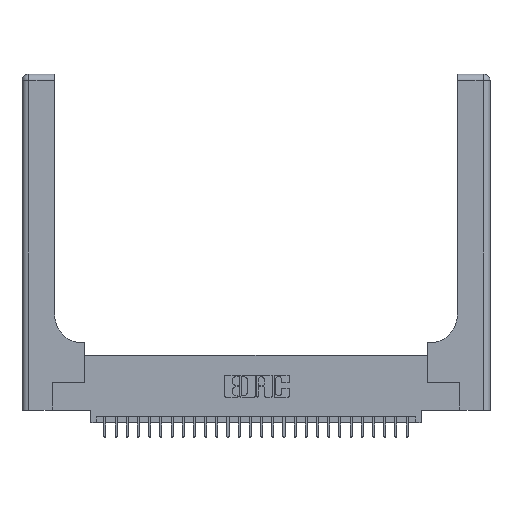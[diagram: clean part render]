
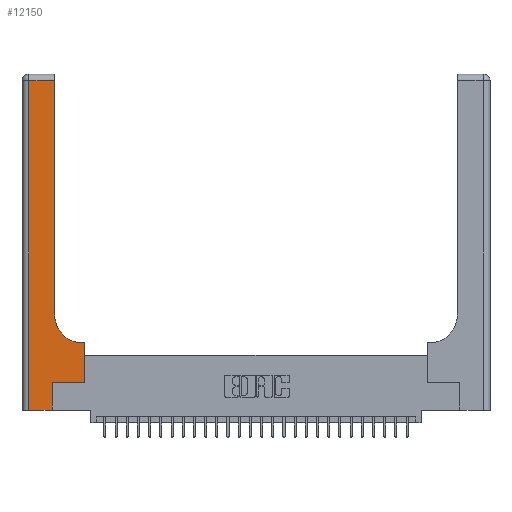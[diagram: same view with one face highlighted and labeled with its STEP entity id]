
A CAD part, top view. The second image highlights one B-rep face of the part: STEP entity #12150.
In plain terms, the highlighted planar face has unit normal (0, 0, 1).
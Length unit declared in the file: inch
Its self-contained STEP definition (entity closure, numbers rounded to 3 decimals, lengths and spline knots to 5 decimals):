
#616 = VECTOR ( 'NONE', #13172, 39.37008 ) ;
#1050 = CARTESIAN_POINT ( 'NONE',  ( 0.5585, 0.25, 0.37 ) ) ;
#1435 = AXIS2_PLACEMENT_3D ( 'NONE', #8181, #15142, #17243 ) ;
#1780 = FACE_OUTER_BOUND ( 'NONE', #25317, .T. ) ;
#2160 = DIRECTION ( 'NONE',  ( 0., 1., 0. ) ) ;
#2464 = VECTOR ( 'NONE', #2160, 39.37008 ) ;
#3300 = LINE ( 'NONE', #1050, #7181 ) ;
#3573 = CARTESIAN_POINT ( 'NONE',  ( 0.2915, 2.94, 0.37 ) ) ;
#4096 = EDGE_CURVE ( 'NONE', #13927, #12521, #15370, .T. ) ;
#4143 = CARTESIAN_POINT ( 'NONE',  ( 0., 0., 0.37 ) ) ;
#4147 = VECTOR ( 'NONE', #22045, 39.37008 ) ;
#4674 = ORIENTED_EDGE ( 'NONE', *, *, #13537, .T. ) ;
#5529 = EDGE_CURVE ( 'NONE', #14583, #12405, #22468, .T. ) ;
#5566 = ORIENTED_EDGE ( 'NONE', *, *, #5529, .T. ) ;
#5905 = DIRECTION ( 'NONE',  ( 1., 0., 0. ) ) ;
#6314 = CARTESIAN_POINT ( 'NONE',  ( 0.269, 0., 0.37 ) ) ;
#6550 = CIRCLE ( 'NONE', #19799, 0.25 ) ;
#7181 = VECTOR ( 'NONE', #7725, 39.37008 ) ;
#7462 = CARTESIAN_POINT ( 'NONE',  ( 0.06, 2.94, 0.37 ) ) ;
#7725 = DIRECTION ( 'NONE',  ( 0., 1., 0. ) ) ;
#7911 = EDGE_CURVE ( 'NONE', #12521, #24864, #22791, .T. ) ;
#8181 = CARTESIAN_POINT ( 'NONE',  ( 0., 3., 0.37 ) ) ;
#9053 = CARTESIAN_POINT ( 'NONE',  ( 0.5415, 0.6, 0.37 ) ) ;
#10012 = EDGE_CURVE ( 'NONE', #28641, #14583, #15413, .T. ) ;
#10838 = PLANE ( 'NONE',  #1435 ) ;
#10984 = VECTOR ( 'NONE', #22379, 39.37008 ) ;
#10993 = CARTESIAN_POINT ( 'NONE',  ( 0.5585, 0.6, 0.37 ) ) ;
#11011 = VERTEX_POINT ( 'NONE', #22078 ) ;
#11362 = DIRECTION ( 'NONE',  ( -1., 0., 0. ) ) ;
#11471 = VECTOR ( 'NONE', #11362, 39.37008 ) ;
#11525 = CARTESIAN_POINT ( 'NONE',  ( 0.2915, 3., 0.37 ) ) ;
#12150 = ADVANCED_FACE ( 'NONE', ( #1780 ), #10838, .F. ) ;
#12405 = VERTEX_POINT ( 'NONE', #23147 ) ;
#12521 = VERTEX_POINT ( 'NONE', #3573 ) ;
#12564 = CARTESIAN_POINT ( 'NONE',  ( 0.5415, 0.85, 0.37 ) ) ;
#12639 = ORIENTED_EDGE ( 'NONE', *, *, #16860, .T. ) ;
#13126 = CARTESIAN_POINT ( 'NONE',  ( 0.269, 0.25, 0.37 ) ) ;
#13148 = ORIENTED_EDGE ( 'NONE', *, *, #21760, .T. ) ;
#13172 = DIRECTION ( 'NONE',  ( 1., 0., 0. ) ) ;
#13273 = LINE ( 'NONE', #13126, #4147 ) ;
#13344 = VERTEX_POINT ( 'NONE', #9053 ) ;
#13370 = VERTEX_POINT ( 'NONE', #10993 ) ;
#13537 = EDGE_CURVE ( 'NONE', #11011, #13370, #3300, .T. ) ;
#13927 = VERTEX_POINT ( 'NONE', #29030 ) ;
#14583 = VERTEX_POINT ( 'NONE', #22043 ) ;
#15142 = DIRECTION ( 'NONE',  ( 0., 0., -1. ) ) ;
#15370 = LINE ( 'NONE', #11525, #24630 ) ;
#15413 = LINE ( 'NONE', #4143, #616 ) ;
#15873 = VECTOR ( 'NONE', #18254, 39.37008 ) ;
#16011 = CARTESIAN_POINT ( 'NONE',  ( 0.06, 3., 0.37 ) ) ;
#16860 = EDGE_CURVE ( 'NONE', #13370, #13344, #27652, .T. ) ;
#17243 = DIRECTION ( 'NONE',  ( -1., 0., 0. ) ) ;
#17843 = ORIENTED_EDGE ( 'NONE', *, *, #24388, .T. ) ;
#18054 = CARTESIAN_POINT ( 'NONE',  ( 0., 2.94, 0.37 ) ) ;
#18254 = DIRECTION ( 'NONE',  ( 0., -1., 0. ) ) ;
#19799 = AXIS2_PLACEMENT_3D ( 'NONE', #12564, #21614, #5905 ) ;
#20201 = ORIENTED_EDGE ( 'NONE', *, *, #10012, .T. ) ;
#21292 = CARTESIAN_POINT ( 'NONE',  ( 0.06, 0., 0.37 ) ) ;
#21614 = DIRECTION ( 'NONE',  ( 0., 0., -1. ) ) ;
#21760 = EDGE_CURVE ( 'NONE', #24864, #28641, #25211, .T. ) ;
#22043 = CARTESIAN_POINT ( 'NONE',  ( 0.269, 0., 0.37 ) ) ;
#22045 = DIRECTION ( 'NONE',  ( 1., 0., 0. ) ) ;
#22055 = ORIENTED_EDGE ( 'NONE', *, *, #25785, .T. ) ;
#22078 = CARTESIAN_POINT ( 'NONE',  ( 0.5585, 0.25, 0.37 ) ) ;
#22379 = DIRECTION ( 'NONE',  ( -1., 0., 0. ) ) ;
#22468 = LINE ( 'NONE', #6314, #2464 ) ;
#22791 = LINE ( 'NONE', #18054, #11471 ) ;
#23147 = CARTESIAN_POINT ( 'NONE',  ( 0.269, 0.25, 0.37 ) ) ;
#24388 = EDGE_CURVE ( 'NONE', #12405, #11011, #13273, .T. ) ;
#24389 = DIRECTION ( 'NONE',  ( 0., 1., 0. ) ) ;
#24630 = VECTOR ( 'NONE', #24389, 39.37008 ) ;
#24864 = VERTEX_POINT ( 'NONE', #7462 ) ;
#25211 = LINE ( 'NONE', #16011, #15873 ) ;
#25317 = EDGE_LOOP ( 'NONE', ( #26406, #28184, #13148, #20201, #5566, #17843, #4674, #12639, #22055 ) ) ;
#25785 = EDGE_CURVE ( 'NONE', #13344, #13927, #6550, .T. ) ;
#26406 = ORIENTED_EDGE ( 'NONE', *, *, #4096, .T. ) ;
#27095 = CARTESIAN_POINT ( 'NONE',  ( 0.2915, 0.6, 0.37 ) ) ;
#27652 = LINE ( 'NONE', #27095, #10984 ) ;
#28184 = ORIENTED_EDGE ( 'NONE', *, *, #7911, .T. ) ;
#28641 = VERTEX_POINT ( 'NONE', #21292 ) ;
#29030 = CARTESIAN_POINT ( 'NONE',  ( 0.2915, 0.85, 0.37 ) ) ;
